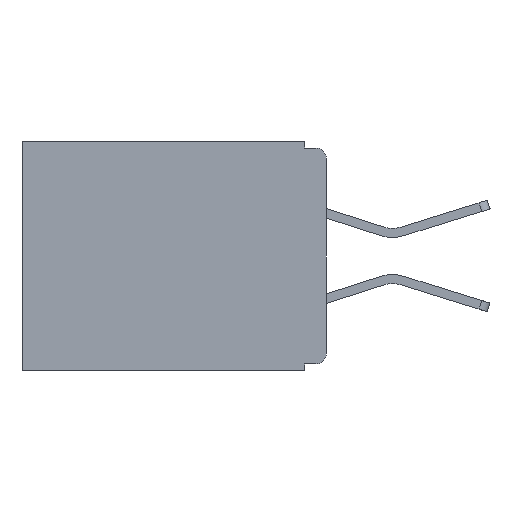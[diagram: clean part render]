
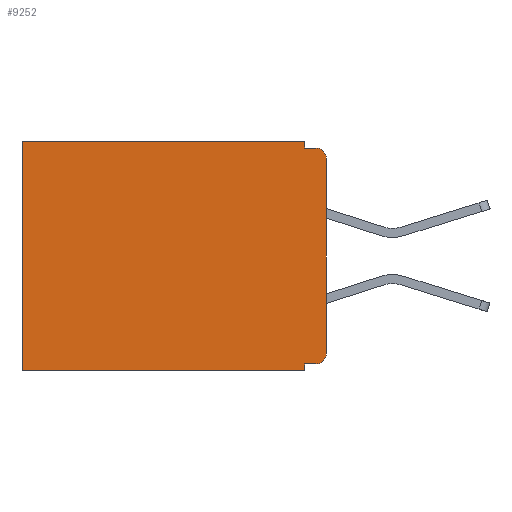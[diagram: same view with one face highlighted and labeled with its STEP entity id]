
A CAD part, left-side view. The second image highlights one B-rep face of the part: STEP entity #9252.
In plain terms, the highlighted planar face has unit normal (-1, 0, 0).
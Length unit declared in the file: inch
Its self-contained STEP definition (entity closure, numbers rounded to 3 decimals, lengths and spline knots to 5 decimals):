
#102 = ORIENTED_EDGE ( 'NONE', *, *, #362, .F. ) ;
#206 = VERTEX_POINT ( 'NONE', #16799 ) ;
#350 = ORIENTED_EDGE ( 'NONE', *, *, #22808, .F. ) ;
#362 = EDGE_CURVE ( 'NONE', #8198, #206, #15681, .T. ) ;
#774 = EDGE_CURVE ( 'NONE', #7222, #24481, #16953, .T. ) ;
#1298 = ORIENTED_EDGE ( 'NONE', *, *, #774, .F. ) ;
#1456 = VECTOR ( 'NONE', #7946, 39.37008 ) ;
#1625 = ORIENTED_EDGE ( 'NONE', *, *, #13518, .T. ) ;
#1710 = ORIENTED_EDGE ( 'NONE', *, *, #23415, .T. ) ;
#1736 = CARTESIAN_POINT ( 'NONE',  ( 0.3, 0., 0. ) ) ;
#1801 = VECTOR ( 'NONE', #10848, 39.37008 ) ;
#2341 = VECTOR ( 'NONE', #18003, 39.37008 ) ;
#2799 = ORIENTED_EDGE ( 'NONE', *, *, #13863, .F. ) ;
#3084 = AXIS2_PLACEMENT_3D ( 'NONE', #14853, #14821, #14804 ) ;
#3296 = ORIENTED_EDGE ( 'NONE', *, *, #22480, .T. ) ;
#3386 = CIRCLE ( 'NONE', #14350, 0.015 ) ;
#4861 = CARTESIAN_POINT ( 'NONE',  ( 0.3, 0.015, -0.025 ) ) ;
#5018 = VECTOR ( 'NONE', #7922, 39.37008 ) ;
#5022 = ORIENTED_EDGE ( 'NONE', *, *, #12953, .F. ) ;
#5172 = CARTESIAN_POINT ( 'NONE',  ( 0.3, 0., -0.01 ) ) ;
#5220 = LINE ( 'NONE', #8991, #25761 ) ;
#6815 = EDGE_CURVE ( 'NONE', #23299, #25262, #18410, .T. ) ;
#6899 = DIRECTION ( 'NONE',  ( 0., 0., -1. ) ) ;
#7222 = VERTEX_POINT ( 'NONE', #21897 ) ;
#7922 = DIRECTION ( 'NONE',  ( 0., 1., 0. ) ) ;
#7946 = DIRECTION ( 'NONE',  ( 0., -1., 0. ) ) ;
#8198 = VERTEX_POINT ( 'NONE', #22211 ) ;
#8734 = AXIS2_PLACEMENT_3D ( 'NONE', #17590, #17583, #17553 ) ;
#8767 = EDGE_LOOP ( 'NONE', ( #5022, #1710, #1298, #2799, #3296, #1625, #11231, #350, #102, #14536 ) ) ;
#8822 = DIRECTION ( 'NONE',  ( 0., 0., -1. ) ) ;
#8899 = VERTEX_POINT ( 'NONE', #25765 ) ;
#8991 = CARTESIAN_POINT ( 'NONE',  ( 0.3, 0.031, 0. ) ) ;
#9252 = ADVANCED_FACE ( 'NONE', ( #22930 ), #17641, .F. ) ;
#9508 = VERTEX_POINT ( 'NONE', #13896 ) ;
#10058 = VECTOR ( 'NONE', #23722, 39.37008 ) ;
#10707 = LINE ( 'NONE', #1736, #10058 ) ;
#10848 = DIRECTION ( 'NONE',  ( 0., 0., -1. ) ) ;
#11005 = VERTEX_POINT ( 'NONE', #17891 ) ;
#11231 = ORIENTED_EDGE ( 'NONE', *, *, #6815, .F. ) ;
#11257 = VECTOR ( 'NONE', #20407, 39.37008 ) ;
#12839 = CARTESIAN_POINT ( 'NONE',  ( 0.3, 0.031, -0.33 ) ) ;
#12953 = EDGE_CURVE ( 'NONE', #20710, #9508, #21866, .T. ) ;
#13392 = EDGE_CURVE ( 'NONE', #8198, #9508, #21238, .T. ) ;
#13518 = EDGE_CURVE ( 'NONE', #8899, #25262, #18786, .T. ) ;
#13600 = CARTESIAN_POINT ( 'NONE',  ( 0.3, 0.437, -0.33 ) ) ;
#13772 = DIRECTION ( 'NONE',  ( 0., 0., -1. ) ) ;
#13863 = EDGE_CURVE ( 'NONE', #11005, #7222, #5220, .T. ) ;
#13896 = CARTESIAN_POINT ( 'NONE',  ( 0.3, 0., -0.305 ) ) ;
#14350 = AXIS2_PLACEMENT_3D ( 'NONE', #4861, #18930, #6899 ) ;
#14536 = ORIENTED_EDGE ( 'NONE', *, *, #13392, .T. ) ;
#14672 = VECTOR ( 'NONE', #13772, 39.37008 ) ;
#14804 = DIRECTION ( 'NONE',  ( 0., 0., -1. ) ) ;
#14821 = DIRECTION ( 'NONE',  ( -1., 0., 0. ) ) ;
#14853 = CARTESIAN_POINT ( 'NONE',  ( 0.3, 0.015, -0.305 ) ) ;
#15681 = LINE ( 'NONE', #15730, #5018 ) ;
#15730 = CARTESIAN_POINT ( 'NONE',  ( 0.3, 0., -0.32 ) ) ;
#16799 = CARTESIAN_POINT ( 'NONE',  ( 0.3, 0.031, -0.32 ) ) ;
#16953 = LINE ( 'NONE', #5172, #1456 ) ;
#17168 = CARTESIAN_POINT ( 'NONE',  ( 0.3, 0.437, -0.33 ) ) ;
#17553 = DIRECTION ( 'NONE',  ( 0., 0., -1. ) ) ;
#17583 = DIRECTION ( 'NONE',  ( 1., 0., 0. ) ) ;
#17590 = CARTESIAN_POINT ( 'NONE',  ( 0.3, 0., -0.33 ) ) ;
#17641 = PLANE ( 'NONE',  #8734 ) ;
#17891 = CARTESIAN_POINT ( 'NONE',  ( 0.3, 0.031, 0. ) ) ;
#17898 = LINE ( 'NONE', #12839, #1801 ) ;
#18003 = DIRECTION ( 'NONE',  ( 0., 1., 0. ) ) ;
#18028 = CARTESIAN_POINT ( 'NONE',  ( 0.3, 0., -0.33 ) ) ;
#18410 = LINE ( 'NONE', #18028, #2341 ) ;
#18786 = LINE ( 'NONE', #13600, #14672 ) ;
#18930 = DIRECTION ( 'NONE',  ( -1., 0., 0. ) ) ;
#20172 = CARTESIAN_POINT ( 'NONE',  ( 0.3, 0.015, -0.01 ) ) ;
#20407 = DIRECTION ( 'NONE',  ( 0., 0., -1. ) ) ;
#20548 = CARTESIAN_POINT ( 'NONE',  ( 0.3, 0.031, -0.33 ) ) ;
#20703 = CARTESIAN_POINT ( 'NONE',  ( 0.3, 0., -0.33 ) ) ;
#20710 = VERTEX_POINT ( 'NONE', #23714 ) ;
#21238 = CIRCLE ( 'NONE', #3084, 0.015 ) ;
#21866 = LINE ( 'NONE', #20703, #11257 ) ;
#21897 = CARTESIAN_POINT ( 'NONE',  ( 0.3, 0.031, -0.01 ) ) ;
#22211 = CARTESIAN_POINT ( 'NONE',  ( 0.3, 0.015, -0.32 ) ) ;
#22480 = EDGE_CURVE ( 'NONE', #11005, #8899, #10707, .T. ) ;
#22808 = EDGE_CURVE ( 'NONE', #206, #23299, #17898, .T. ) ;
#22930 = FACE_OUTER_BOUND ( 'NONE', #8767, .T. ) ;
#23299 = VERTEX_POINT ( 'NONE', #20548 ) ;
#23415 = EDGE_CURVE ( 'NONE', #20710, #24481, #3386, .T. ) ;
#23714 = CARTESIAN_POINT ( 'NONE',  ( 0.3, 0., -0.025 ) ) ;
#23722 = DIRECTION ( 'NONE',  ( 0., 1., 0. ) ) ;
#24481 = VERTEX_POINT ( 'NONE', #20172 ) ;
#25262 = VERTEX_POINT ( 'NONE', #17168 ) ;
#25761 = VECTOR ( 'NONE', #8822, 39.37008 ) ;
#25765 = CARTESIAN_POINT ( 'NONE',  ( 0.3, 0.437, 0. ) ) ;
